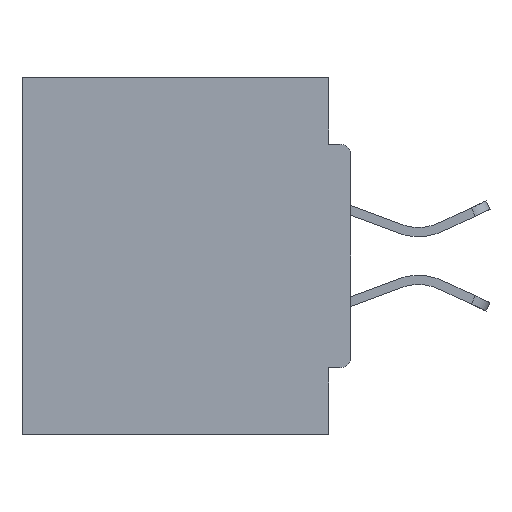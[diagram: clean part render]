
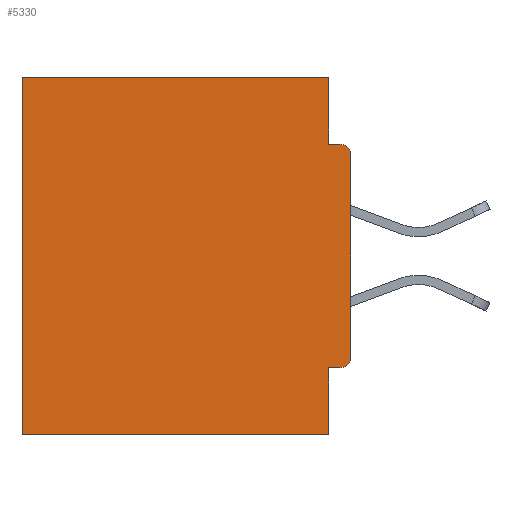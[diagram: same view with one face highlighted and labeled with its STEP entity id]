
A CAD part, left-side view. The second image highlights one B-rep face of the part: STEP entity #5330.
In plain terms, the highlighted planar face has unit normal (-1, 0, 0).
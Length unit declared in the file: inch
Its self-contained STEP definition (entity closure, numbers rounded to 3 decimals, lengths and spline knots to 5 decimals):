
#1097 = EDGE_LOOP ( 'NONE', ( #11399, #21155, #25101, #8961, #22090, #30323, #15739, #2677, #24893, #18396 ) ) ;
#1428 = CIRCLE ( 'NONE', #29438, 0.015 ) ;
#1526 = LINE ( 'NONE', #23465, #17910 ) ;
#1638 = AXIS2_PLACEMENT_3D ( 'NONE', #34980, #10068, #32044 ) ;
#1769 = DIRECTION ( 'NONE',  ( 1., 0., 0. ) ) ;
#1905 = DIRECTION ( 'NONE',  ( 0., 0., -1. ) ) ;
#2215 = LINE ( 'NONE', #34472, #25073 ) ;
#2482 = EDGE_CURVE ( 'NONE', #2978, #22192, #19397, .T. ) ;
#2677 = ORIENTED_EDGE ( 'NONE', *, *, #2482, .F. ) ;
#2978 = VERTEX_POINT ( 'NONE', #25097 ) ;
#3761 = VECTOR ( 'NONE', #10777, 39.37008 ) ;
#4165 = VECTOR ( 'NONE', #17298, 39.37008 ) ;
#4558 = EDGE_CURVE ( 'NONE', #22192, #11745, #11110, .T. ) ;
#4846 = CARTESIAN_POINT ( 'NONE',  ( 0.298, 0.015, -0.3915 ) ) ;
#5051 = CARTESIAN_POINT ( 'NONE',  ( 0.298, 0.46, 0. ) ) ;
#5104 = DIRECTION ( 'NONE',  ( 0., 0., -1. ) ) ;
#5175 = EDGE_CURVE ( 'NONE', #27507, #8519, #1526, .T. ) ;
#5330 = ADVANCED_FACE ( 'NONE', ( #11033 ), #26970, .F. ) ;
#5555 = VECTOR ( 'NONE', #14110, 39.37008 ) ;
#6942 = CARTESIAN_POINT ( 'NONE',  ( 0.298, 0.031, -0.5 ) ) ;
#7096 = CARTESIAN_POINT ( 'NONE',  ( 0.298, 0.015, -0.0935 ) ) ;
#7882 = EDGE_CURVE ( 'NONE', #15717, #27507, #27917, .T. ) ;
#7996 = VERTEX_POINT ( 'NONE', #5051 ) ;
#8519 = VERTEX_POINT ( 'NONE', #7096 ) ;
#8961 = ORIENTED_EDGE ( 'NONE', *, *, #22089, .T. ) ;
#10068 = DIRECTION ( 'NONE',  ( -1., 0., 0. ) ) ;
#10334 = CARTESIAN_POINT ( 'NONE',  ( 0.298, 0., 0. ) ) ;
#10350 = CARTESIAN_POINT ( 'NONE',  ( 0.298, 0.031, 0. ) ) ;
#10568 = DIRECTION ( 'NONE',  ( 0., 0., -1. ) ) ;
#10777 = DIRECTION ( 'NONE',  ( 0., 0., -1. ) ) ;
#11033 = FACE_OUTER_BOUND ( 'NONE', #1097, .T. ) ;
#11099 = EDGE_CURVE ( 'NONE', #28688, #18808, #28996, .T. ) ;
#11110 = LINE ( 'NONE', #24508, #3761 ) ;
#11399 = ORIENTED_EDGE ( 'NONE', *, *, #33010, .T. ) ;
#11494 = LINE ( 'NONE', #23224, #4165 ) ;
#11745 = VERTEX_POINT ( 'NONE', #12714 ) ;
#11755 = DIRECTION ( 'NONE',  ( 0., 1., 0. ) ) ;
#12568 = VECTOR ( 'NONE', #16579, 39.37008 ) ;
#12714 = CARTESIAN_POINT ( 'NONE',  ( 0.298, 0.031, -0.5 ) ) ;
#13228 = VECTOR ( 'NONE', #1905, 39.37008 ) ;
#13325 = CARTESIAN_POINT ( 'NONE',  ( 0.298, 0., -0.3915 ) ) ;
#13796 = CARTESIAN_POINT ( 'NONE',  ( 0.298, 0., 0. ) ) ;
#14110 = DIRECTION ( 'NONE',  ( 0., 0., -1. ) ) ;
#15119 = DIRECTION ( 'NONE',  ( 0., -1., 0. ) ) ;
#15717 = VERTEX_POINT ( 'NONE', #10350 ) ;
#15739 = ORIENTED_EDGE ( 'NONE', *, *, #4558, .F. ) ;
#15752 = VERTEX_POINT ( 'NONE', #34777 ) ;
#16130 = EDGE_CURVE ( 'NONE', #7996, #15752, #18904, .T. ) ;
#16372 = VECTOR ( 'NONE', #11755, 39.37008 ) ;
#16579 = DIRECTION ( 'NONE',  ( 0., 0., -1. ) ) ;
#17298 = DIRECTION ( 'NONE',  ( 0., 1., 0. ) ) ;
#17910 = VECTOR ( 'NONE', #15119, 39.37008 ) ;
#18396 = ORIENTED_EDGE ( 'NONE', *, *, #11099, .F. ) ;
#18808 = VERTEX_POINT ( 'NONE', #13325 ) ;
#18904 = LINE ( 'NONE', #30685, #5555 ) ;
#19381 = EDGE_CURVE ( 'NONE', #11745, #15752, #11494, .T. ) ;
#19397 = LINE ( 'NONE', #23096, #16372 ) ;
#21155 = ORIENTED_EDGE ( 'NONE', *, *, #5175, .F. ) ;
#22089 = EDGE_CURVE ( 'NONE', #15717, #7996, #2215, .T. ) ;
#22090 = ORIENTED_EDGE ( 'NONE', *, *, #16130, .T. ) ;
#22192 = VERTEX_POINT ( 'NONE', #35752 ) ;
#23096 = CARTESIAN_POINT ( 'NONE',  ( 0.298, 0., -0.4065 ) ) ;
#23224 = CARTESIAN_POINT ( 'NONE',  ( 0.298, 0., -0.5 ) ) ;
#23465 = CARTESIAN_POINT ( 'NONE',  ( 0.298, 0., -0.0935 ) ) ;
#24508 = CARTESIAN_POINT ( 'NONE',  ( 0.298, 0.031, -0.5 ) ) ;
#24893 = ORIENTED_EDGE ( 'NONE', *, *, #25081, .T. ) ;
#25073 = VECTOR ( 'NONE', #26315, 39.37008 ) ;
#25081 = EDGE_CURVE ( 'NONE', #2978, #18808, #1428, .T. ) ;
#25097 = CARTESIAN_POINT ( 'NONE',  ( 0.298, 0.015, -0.4065 ) ) ;
#25101 = ORIENTED_EDGE ( 'NONE', *, *, #7882, .F. ) ;
#26315 = DIRECTION ( 'NONE',  ( 0., 1., 0. ) ) ;
#26970 = PLANE ( 'NONE',  #33003 ) ;
#27507 = VERTEX_POINT ( 'NONE', #27696 ) ;
#27696 = CARTESIAN_POINT ( 'NONE',  ( 0.298, 0.031, -0.0935 ) ) ;
#27917 = LINE ( 'NONE', #6942, #13228 ) ;
#28688 = VERTEX_POINT ( 'NONE', #33029 ) ;
#28996 = LINE ( 'NONE', #13796, #12568 ) ;
#29438 = AXIS2_PLACEMENT_3D ( 'NONE', #4846, #29825, #5104 ) ;
#29825 = DIRECTION ( 'NONE',  ( -1., 0., 0. ) ) ;
#30323 = ORIENTED_EDGE ( 'NONE', *, *, #19381, .F. ) ;
#30685 = CARTESIAN_POINT ( 'NONE',  ( 0.298, 0.46, 0. ) ) ;
#32044 = DIRECTION ( 'NONE',  ( 0., 0., -1. ) ) ;
#33003 = AXIS2_PLACEMENT_3D ( 'NONE', #10334, #1769, #10568 ) ;
#33010 = EDGE_CURVE ( 'NONE', #28688, #8519, #33159, .T. ) ;
#33029 = CARTESIAN_POINT ( 'NONE',  ( 0.298, 0., -0.1085 ) ) ;
#33159 = CIRCLE ( 'NONE', #1638, 0.015 ) ;
#34472 = CARTESIAN_POINT ( 'NONE',  ( 0.298, 0., 0. ) ) ;
#34777 = CARTESIAN_POINT ( 'NONE',  ( 0.298, 0.46, -0.5 ) ) ;
#34980 = CARTESIAN_POINT ( 'NONE',  ( 0.298, 0.015, -0.1085 ) ) ;
#35752 = CARTESIAN_POINT ( 'NONE',  ( 0.298, 0.031, -0.4065 ) ) ;
